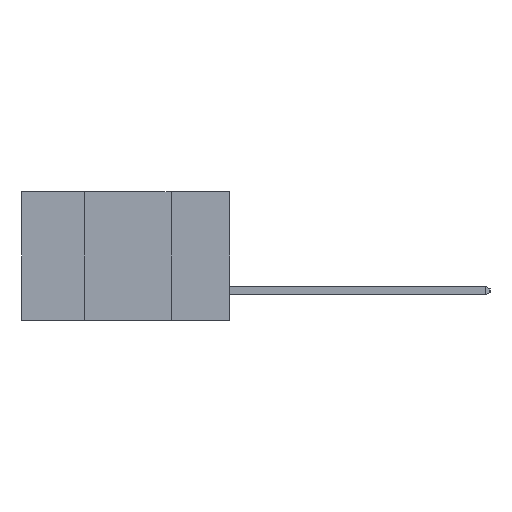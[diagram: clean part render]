
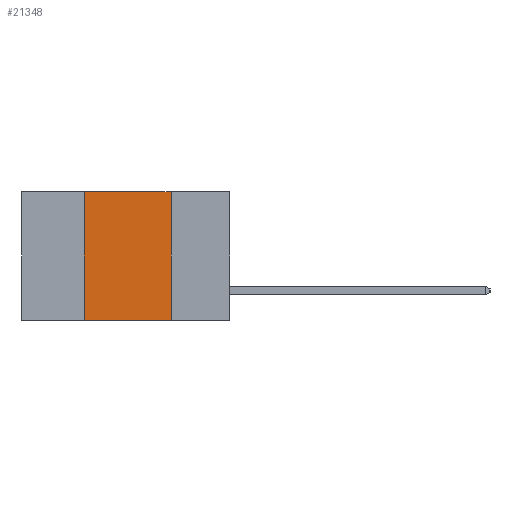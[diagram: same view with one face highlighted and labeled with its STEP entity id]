
A CAD part, left-side view. The second image highlights one B-rep face of the part: STEP entity #21348.
In plain terms, the highlighted planar face has unit normal (-1, 0, 0).
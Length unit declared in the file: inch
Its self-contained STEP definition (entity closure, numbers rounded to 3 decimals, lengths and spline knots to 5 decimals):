
#1 = VECTOR ( 'NONE', #15767, 39.37008 ) ;
#1730 = VECTOR ( 'NONE', #20466, 39.37008 ) ;
#2368 = FACE_OUTER_BOUND ( 'NONE', #9335, .T. ) ;
#2431 = CARTESIAN_POINT ( 'NONE',  ( 0., 0.17, -0.37 ) ) ;
#3437 = CARTESIAN_POINT ( 'NONE',  ( 0., 0.6, 0. ) ) ;
#3831 = ORIENTED_EDGE ( 'NONE', *, *, #9373, .F. ) ;
#4220 = VERTEX_POINT ( 'NONE', #5925 ) ;
#5267 = EDGE_CURVE ( 'NONE', #22952, #4220, #8897, .T. ) ;
#5765 = DIRECTION ( 'NONE',  ( 0., 0., -1. ) ) ;
#5925 = CARTESIAN_POINT ( 'NONE',  ( 0., 0.17, 0. ) ) ;
#6167 = LINE ( 'NONE', #6434, #1 ) ;
#6434 = CARTESIAN_POINT ( 'NONE',  ( 0., 0.6, -0.37 ) ) ;
#7798 = VERTEX_POINT ( 'NONE', #2431 ) ;
#8897 = LINE ( 'NONE', #14755, #20537 ) ;
#9217 = VECTOR ( 'NONE', #16592, 39.37008 ) ;
#9335 = EDGE_LOOP ( 'NONE', ( #23084, #12885, #3831, #20171 ) ) ;
#9373 = EDGE_CURVE ( 'NONE', #17176, #22952, #18137, .T. ) ;
#11171 = CARTESIAN_POINT ( 'NONE',  ( 0., 0.42, 0. ) ) ;
#12885 = ORIENTED_EDGE ( 'NONE', *, *, #5267, .F. ) ;
#14234 = CARTESIAN_POINT ( 'NONE',  ( 0., 0.17, 0. ) ) ;
#14755 = CARTESIAN_POINT ( 'NONE',  ( 0., 0.6, 0. ) ) ;
#15767 = DIRECTION ( 'NONE',  ( 0., -1., 0. ) ) ;
#16592 = DIRECTION ( 'NONE',  ( 0., 0., -1. ) ) ;
#17176 = VERTEX_POINT ( 'NONE', #18978 ) ;
#18137 = LINE ( 'NONE', #11171, #1730 ) ;
#18732 = EDGE_CURVE ( 'NONE', #17176, #7798, #6167, .T. ) ;
#18978 = CARTESIAN_POINT ( 'NONE',  ( 0., 0.42, -0.37 ) ) ;
#19740 = DIRECTION ( 'NONE',  ( 1., 0., 0. ) ) ;
#20171 = ORIENTED_EDGE ( 'NONE', *, *, #18732, .T. ) ;
#20466 = DIRECTION ( 'NONE',  ( 0., 0., 1. ) ) ;
#20537 = VECTOR ( 'NONE', #28629, 39.37008 ) ;
#20891 = AXIS2_PLACEMENT_3D ( 'NONE', #3437, #19740, #5765 ) ;
#21348 = ADVANCED_FACE ( 'NONE', ( #2368 ), #26608, .F. ) ;
#21827 = EDGE_CURVE ( 'NONE', #4220, #7798, #28461, .T. ) ;
#22952 = VERTEX_POINT ( 'NONE', #24391 ) ;
#23084 = ORIENTED_EDGE ( 'NONE', *, *, #21827, .F. ) ;
#24391 = CARTESIAN_POINT ( 'NONE',  ( 0., 0.42, 0. ) ) ;
#26608 = PLANE ( 'NONE',  #20891 ) ;
#28461 = LINE ( 'NONE', #14234, #9217 ) ;
#28629 = DIRECTION ( 'NONE',  ( 0., -1., 0. ) ) ;
